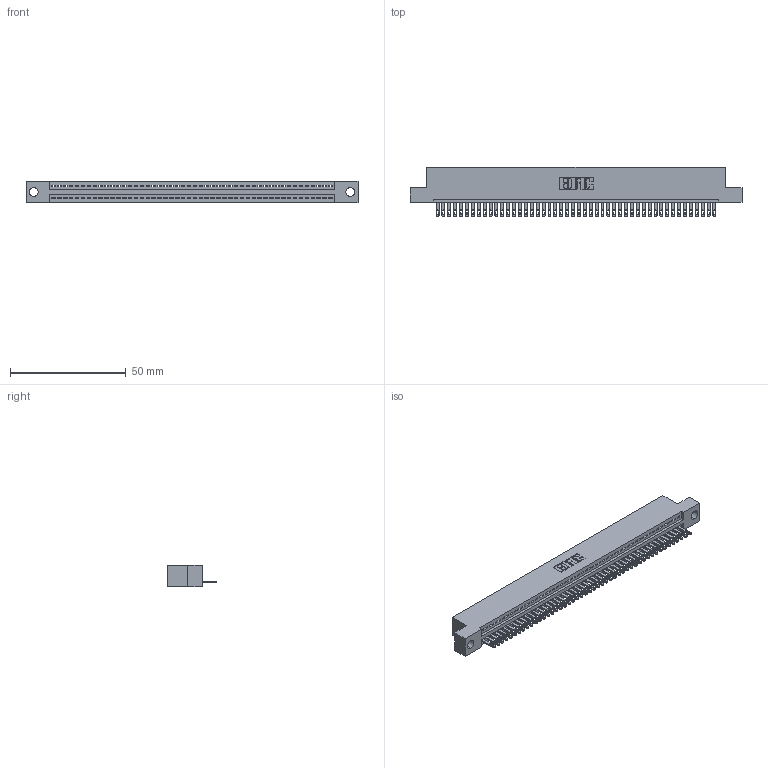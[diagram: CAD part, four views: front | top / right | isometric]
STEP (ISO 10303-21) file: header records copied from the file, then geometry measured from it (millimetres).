
FILE_DESCRIPTION (( 'STEP AP203' ), '1' );
FILE_NAME ('345-048-500-104.STEP', '2019-10-09T03:44:31', ( '' ), ( '' ), 'SwSTEP 2.0', 'SolidWorks 2016', '' );
FILE_SCHEMA (( 'CONFIG_CONTROL_DESIGN' ));
Length unit declared in the file: inch
Products named in the file (3): 345-048-500-104; 345-292-001_345-293-100; 345 Part_Flush Mounting Lugs - 0.156 Dia-TH
Assembly tree (49 placements, depth 2):
  345-048-500-104
    345 Part_Flush Mounting Lugs - 0.156 Dia-TH
    345-292-001_345-293-100  x48
Bounding box: 143.13 x 21.51 x 9.4 mm (x, y, z)
Volume: 13585.5 mm3; surface area: 18052.1 mm2
Topology: 49 solids, 49 shells, 2718 faces, 8405 edges, 5602 vertices
Faces by surface type: plane 1712, cylinder 1006
Entity records: 35251 total; most frequent: CARTESIAN_POINT 6112, ORIENTED_EDGE 6094, DIRECTION 5331, EDGE_CURVE 3047, VECTOR 2719, LINE 2719, VERTEX_POINT 2030, AXIS2_PLACEMENT_3D 1306
